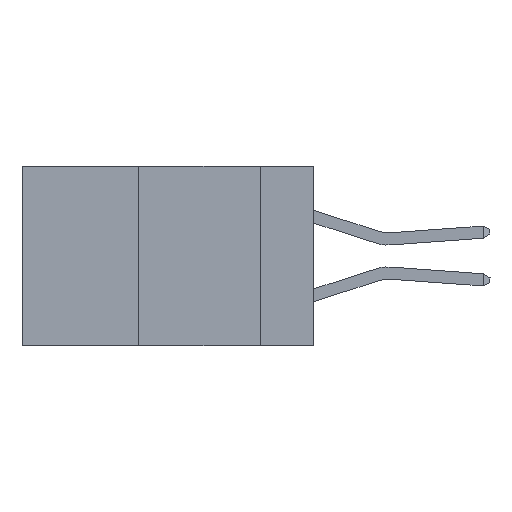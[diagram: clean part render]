
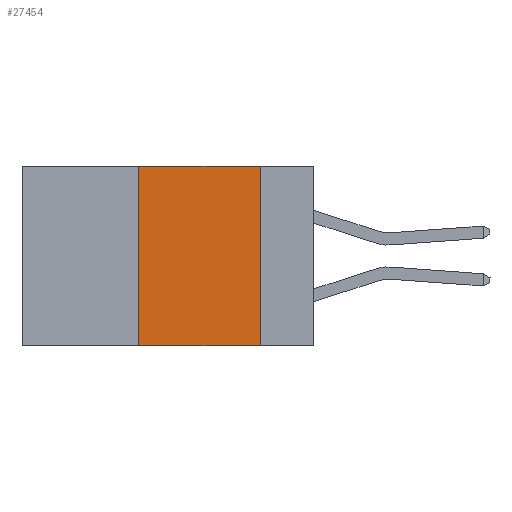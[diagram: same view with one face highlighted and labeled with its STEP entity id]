
A CAD part, left-side view. The second image highlights one B-rep face of the part: STEP entity #27454.
In plain terms, the highlighted planar face has unit normal (-1, 0, 0).
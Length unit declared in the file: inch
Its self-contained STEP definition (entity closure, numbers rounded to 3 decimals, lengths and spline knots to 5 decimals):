
#970 = VECTOR ( 'NONE', #27415, 39.37008 ) ;
#2656 = EDGE_LOOP ( 'NONE', ( #9139, #21021, #31174, #21354 ) ) ;
#2732 = LINE ( 'NONE', #29635, #30432 ) ;
#5801 = VECTOR ( 'NONE', #13072, 39.37008 ) ;
#6475 = EDGE_CURVE ( 'NONE', #23837, #28594, #13087, .T. ) ;
#7165 = CARTESIAN_POINT ( 'NONE',  ( 0., 0.6, 0. ) ) ;
#8436 = LINE ( 'NONE', #13288, #970 ) ;
#9139 = ORIENTED_EDGE ( 'NONE', *, *, #18867, .F. ) ;
#9357 = FACE_OUTER_BOUND ( 'NONE', #2656, .T. ) ;
#9440 = EDGE_CURVE ( 'NONE', #33236, #24145, #16795, .T. ) ;
#11694 = DIRECTION ( 'NONE',  ( 0., 0., -1. ) ) ;
#13072 = DIRECTION ( 'NONE',  ( 0., -1., 0. ) ) ;
#13087 = LINE ( 'NONE', #23007, #25867 ) ;
#13288 = CARTESIAN_POINT ( 'NONE',  ( 0., 0.11, 0. ) ) ;
#13324 = CARTESIAN_POINT ( 'NONE',  ( 0., 0.11, -0.37 ) ) ;
#14965 = EDGE_CURVE ( 'NONE', #23837, #33236, #2732, .T. ) ;
#15619 = DIRECTION ( 'NONE',  ( 0., 0., 1. ) ) ;
#16795 = LINE ( 'NONE', #7165, #5801 ) ;
#17208 = DIRECTION ( 'NONE',  ( 1., 0., 0. ) ) ;
#18867 = EDGE_CURVE ( 'NONE', #24145, #28594, #8436, .T. ) ;
#20478 = CARTESIAN_POINT ( 'NONE',  ( 0., 0.36, -0.37 ) ) ;
#21021 = ORIENTED_EDGE ( 'NONE', *, *, #9440, .F. ) ;
#21223 = AXIS2_PLACEMENT_3D ( 'NONE', #34076, #17208, #11694 ) ;
#21354 = ORIENTED_EDGE ( 'NONE', *, *, #6475, .T. ) ;
#23007 = CARTESIAN_POINT ( 'NONE',  ( 0., 0.6, -0.37 ) ) ;
#23837 = VERTEX_POINT ( 'NONE', #20478 ) ;
#24145 = VERTEX_POINT ( 'NONE', #25225 ) ;
#25225 = CARTESIAN_POINT ( 'NONE',  ( 0., 0.11, 0. ) ) ;
#25867 = VECTOR ( 'NONE', #26182, 39.37008 ) ;
#26182 = DIRECTION ( 'NONE',  ( 0., -1., 0. ) ) ;
#27415 = DIRECTION ( 'NONE',  ( 0., 0., -1. ) ) ;
#27454 = ADVANCED_FACE ( 'NONE', ( #9357 ), #28517, .F. ) ;
#28517 = PLANE ( 'NONE',  #21223 ) ;
#28594 = VERTEX_POINT ( 'NONE', #13324 ) ;
#29635 = CARTESIAN_POINT ( 'NONE',  ( 0., 0.36, 0. ) ) ;
#30432 = VECTOR ( 'NONE', #15619, 39.37008 ) ;
#31174 = ORIENTED_EDGE ( 'NONE', *, *, #14965, .F. ) ;
#33236 = VERTEX_POINT ( 'NONE', #33805 ) ;
#33805 = CARTESIAN_POINT ( 'NONE',  ( 0., 0.36, 0. ) ) ;
#34076 = CARTESIAN_POINT ( 'NONE',  ( 0., 0.6, 0. ) ) ;
